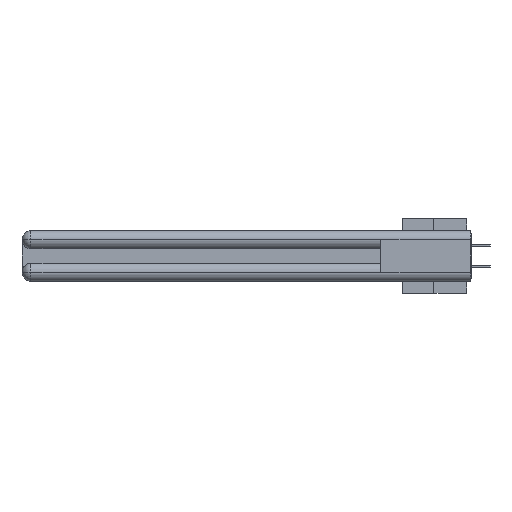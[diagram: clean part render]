
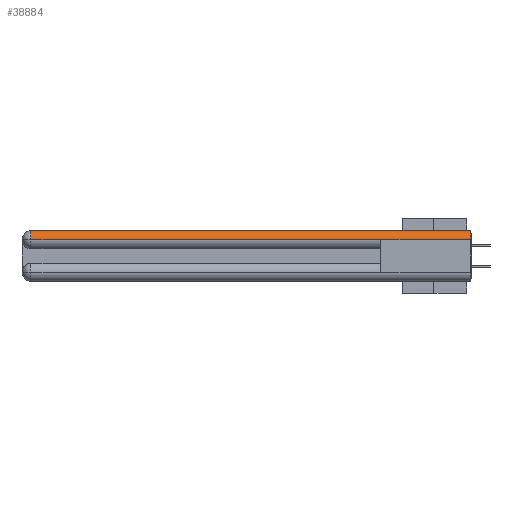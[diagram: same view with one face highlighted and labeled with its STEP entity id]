
A CAD part, left-side view. The second image highlights one B-rep face of the part: STEP entity #38884.
In plain terms, the highlighted cylindrical face has radius 1.562 mm (diameter 3.124 mm), a partial arc.
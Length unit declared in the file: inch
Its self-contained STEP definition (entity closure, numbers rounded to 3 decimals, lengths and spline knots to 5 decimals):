
#676 = DIRECTION ( 'NONE',  ( 0., -1., 0. ) ) ;
#1167 = EDGE_LOOP ( 'NONE', ( #23552, #30657, #21356, #3425, #29972 ) ) ;
#2665 = EDGE_CURVE ( 'NONE', #27707, #17211, #12341, .T. ) ;
#3407 = AXIS2_PLACEMENT_3D ( 'NONE', #14563, #8156, #37647 ) ;
#3425 = ORIENTED_EDGE ( 'NONE', *, *, #32703, .F. ) ;
#3979 = DIRECTION ( 'NONE',  ( 0., -1., 0. ) ) ;
#5638 = VERTEX_POINT ( 'NONE', #23302 ) ;
#5921 = CIRCLE ( 'NONE', #3407, 0.0615 ) ;
#5965 = CARTESIAN_POINT ( 'NONE',  ( 0., 2.94, -0.0615 ) ) ;
#6379 = FACE_OUTER_BOUND ( 'NONE', #1167, .T. ) ;
#8156 = DIRECTION ( 'NONE',  ( 0., -1., 0. ) ) ;
#12341 = LINE ( 'NONE', #26676, #19451 ) ;
#13981 = VERTEX_POINT ( 'NONE', #19065 ) ;
#14563 = CARTESIAN_POINT ( 'NONE',  ( 0.0615, 2.94, -0.0615 ) ) ;
#14716 = AXIS2_PLACEMENT_3D ( 'NONE', #38609, #28327, #38192 ) ;
#14746 = LINE ( 'NONE', #20160, #40805 ) ;
#16364 = DIRECTION ( 'NONE',  ( 1., 0., 0. ) ) ;
#16986 = VERTEX_POINT ( 'NONE', #5965 ) ;
#17211 = VERTEX_POINT ( 'NONE', #19733 ) ;
#17945 = VECTOR ( 'NONE', #28261, 39.37008 ) ;
#18008 = CARTESIAN_POINT ( 'NONE',  ( 0.0615, 2.94, 0. ) ) ;
#19065 = CARTESIAN_POINT ( 'NONE',  ( 0., 0., -0.0615 ) ) ;
#19451 = VECTOR ( 'NONE', #36238, 39.37008 ) ;
#19641 = CIRCLE ( 'NONE', #31740, 0.0615 ) ;
#19733 = CARTESIAN_POINT ( 'NONE',  ( 0.0615, 0., 0. ) ) ;
#20160 = CARTESIAN_POINT ( 'NONE',  ( 0., 3., -0.0615 ) ) ;
#21356 = ORIENTED_EDGE ( 'NONE', *, *, #28682, .T. ) ;
#22041 = EDGE_CURVE ( 'NONE', #27707, #16986, #5921, .T. ) ;
#22292 = EDGE_CURVE ( 'NONE', #17211, #13981, #19641, .T. ) ;
#22514 = LINE ( 'NONE', #37990, #17945 ) ;
#22670 = CYLINDRICAL_SURFACE ( 'NONE', #14716, 0.0615 ) ;
#23302 = CARTESIAN_POINT ( 'NONE',  ( 0., 0.6, -0.0615 ) ) ;
#23552 = ORIENTED_EDGE ( 'NONE', *, *, #2665, .F. ) ;
#26676 = CARTESIAN_POINT ( 'NONE',  ( 0.0615, 0., 0. ) ) ;
#27707 = VERTEX_POINT ( 'NONE', #18008 ) ;
#28261 = DIRECTION ( 'NONE',  ( 0., 1., 0. ) ) ;
#28327 = DIRECTION ( 'NONE',  ( 0., 1., 0. ) ) ;
#28682 = EDGE_CURVE ( 'NONE', #16986, #5638, #14746, .T. ) ;
#29972 = ORIENTED_EDGE ( 'NONE', *, *, #22292, .F. ) ;
#30657 = ORIENTED_EDGE ( 'NONE', *, *, #22041, .T. ) ;
#31740 = AXIS2_PLACEMENT_3D ( 'NONE', #33031, #3979, #16364 ) ;
#32703 = EDGE_CURVE ( 'NONE', #13981, #5638, #22514, .T. ) ;
#33031 = CARTESIAN_POINT ( 'NONE',  ( 0.0615, 0., -0.0615 ) ) ;
#36238 = DIRECTION ( 'NONE',  ( 0., -1., 0. ) ) ;
#37647 = DIRECTION ( 'NONE',  ( 0., 0., 1. ) ) ;
#37990 = CARTESIAN_POINT ( 'NONE',  ( 0., 3., -0.0615 ) ) ;
#38192 = DIRECTION ( 'NONE',  ( 0., 0., 1. ) ) ;
#38609 = CARTESIAN_POINT ( 'NONE',  ( 0.0615, 0., -0.0615 ) ) ;
#38884 = ADVANCED_FACE ( 'NONE', ( #6379 ), #22670, .T. ) ;
#40805 = VECTOR ( 'NONE', #676, 39.37008 ) ;
